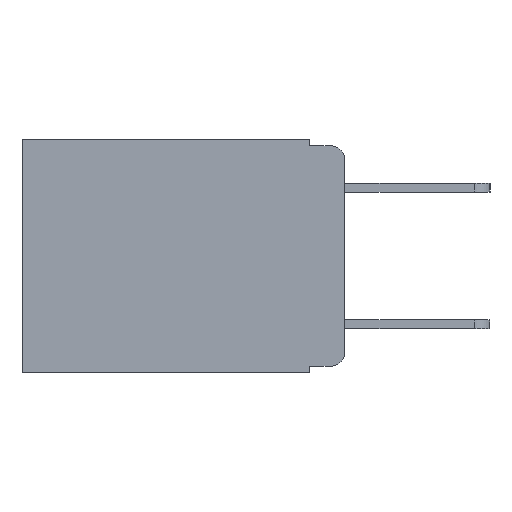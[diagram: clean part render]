
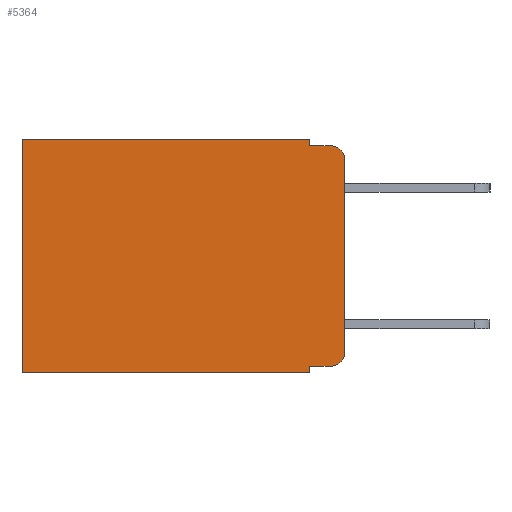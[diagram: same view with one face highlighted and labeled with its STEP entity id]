
A CAD part, left-side view. The second image highlights one B-rep face of the part: STEP entity #5364.
In plain terms, the highlighted planar face has unit normal (-1, 0, 0).
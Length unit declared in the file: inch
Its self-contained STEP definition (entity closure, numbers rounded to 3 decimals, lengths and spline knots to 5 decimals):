
#39 = CARTESIAN_POINT ( 'NONE',  ( 0.298, 0.02, -0.03 ) ) ;
#48 = DIRECTION ( 'NONE',  ( 0., 0., -1. ) ) ;
#63 = VECTOR ( 'NONE', #7219, 39.37008 ) ;
#110 = CARTESIAN_POINT ( 'NONE',  ( 0.298, 0.051, 0. ) ) ;
#261 = ORIENTED_EDGE ( 'NONE', *, *, #4101, .T. ) ;
#610 = CARTESIAN_POINT ( 'NONE',  ( 0.298, 0.051, 0. ) ) ;
#1132 = EDGE_CURVE ( 'NONE', #8445, #1394, #11662, .T. ) ;
#1369 = VERTEX_POINT ( 'NONE', #3259 ) ;
#1370 = EDGE_CURVE ( 'NONE', #6006, #1394, #7896, .T. ) ;
#1394 = VERTEX_POINT ( 'NONE', #6866 ) ;
#1484 = LINE ( 'NONE', #9484, #6356 ) ;
#1754 = CARTESIAN_POINT ( 'NONE',  ( 0.298, 0.051, -0.333 ) ) ;
#1926 = CARTESIAN_POINT ( 'NONE',  ( 0.298, 0., -0.03 ) ) ;
#1969 = DIRECTION ( 'NONE',  ( -1., 0., 0. ) ) ;
#2356 = VERTEX_POINT ( 'NONE', #8151 ) ;
#2420 = DIRECTION ( 'NONE',  ( 0., 0., -1. ) ) ;
#2481 = CARTESIAN_POINT ( 'NONE',  ( 0.298, 0.051, -0.333 ) ) ;
#2482 = DIRECTION ( 'NONE',  ( 0., 0., -1. ) ) ;
#2542 = DIRECTION ( 'NONE',  ( 0., 0., -1. ) ) ;
#2548 = CARTESIAN_POINT ( 'NONE',  ( 0.298, 0.051, -0.343 ) ) ;
#2586 = AXIS2_PLACEMENT_3D ( 'NONE', #3926, #7556, #2420 ) ;
#2650 = DIRECTION ( 'NONE',  ( 0., 0., -1. ) ) ;
#2749 = EDGE_LOOP ( 'NONE', ( #3449, #7786, #8917, #2861, #9144, #10350, #8103, #8748, #261, #3269 ) ) ;
#2774 = CARTESIAN_POINT ( 'NONE',  ( 0.298, 0.473, 0. ) ) ;
#2861 = ORIENTED_EDGE ( 'NONE', *, *, #6523, .F. ) ;
#3032 = CARTESIAN_POINT ( 'NONE',  ( 0.298, 0.02, -0.313 ) ) ;
#3047 = LINE ( 'NONE', #610, #10782 ) ;
#3259 = CARTESIAN_POINT ( 'NONE',  ( 0.298, 0.02, -0.01 ) ) ;
#3260 = VECTOR ( 'NONE', #10368, 39.37008 ) ;
#3269 = ORIENTED_EDGE ( 'NONE', *, *, #1132, .T. ) ;
#3314 = CARTESIAN_POINT ( 'NONE',  ( 0.298, 0.051, 0. ) ) ;
#3449 = ORIENTED_EDGE ( 'NONE', *, *, #1370, .F. ) ;
#3595 = AXIS2_PLACEMENT_3D ( 'NONE', #39, #1969, #9251 ) ;
#3722 = LINE ( 'NONE', #110, #10952 ) ;
#3926 = CARTESIAN_POINT ( 'NONE',  ( 0.298, 0., 0. ) ) ;
#4101 = EDGE_CURVE ( 'NONE', #10851, #8445, #7963, .T. ) ;
#4497 = LINE ( 'NONE', #11727, #63 ) ;
#4716 = EDGE_CURVE ( 'NONE', #11555, #2356, #4497, .T. ) ;
#4819 = DIRECTION ( 'NONE',  ( 0., 0., -1. ) ) ;
#4927 = EDGE_CURVE ( 'NONE', #7244, #1369, #1484, .T. ) ;
#5047 = CARTESIAN_POINT ( 'NONE',  ( 0.298, 0., 0. ) ) ;
#5228 = FACE_OUTER_BOUND ( 'NONE', #2749, .T. ) ;
#5263 = EDGE_CURVE ( 'NONE', #10851, #11555, #3047, .T. ) ;
#5319 = CIRCLE ( 'NONE', #3595, 0.02 ) ;
#5343 = LINE ( 'NONE', #11486, #8007 ) ;
#5364 = ADVANCED_FACE ( 'NONE', ( #5228 ), #11501, .F. ) ;
#5790 = VECTOR ( 'NONE', #2482, 39.37008 ) ;
#5970 = AXIS2_PLACEMENT_3D ( 'NONE', #3032, #11044, #4819 ) ;
#6006 = VERTEX_POINT ( 'NONE', #1926 ) ;
#6356 = VECTOR ( 'NONE', #8579, 39.37008 ) ;
#6523 = EDGE_CURVE ( 'NONE', #8996, #7244, #3722, .T. ) ;
#6866 = CARTESIAN_POINT ( 'NONE',  ( 0.298, 0., -0.313 ) ) ;
#7219 = DIRECTION ( 'NONE',  ( 0., 1., 0. ) ) ;
#7244 = VERTEX_POINT ( 'NONE', #9757 ) ;
#7556 = DIRECTION ( 'NONE',  ( 1., 0., 0. ) ) ;
#7786 = ORIENTED_EDGE ( 'NONE', *, *, #8191, .T. ) ;
#7896 = LINE ( 'NONE', #5047, #5790 ) ;
#7963 = LINE ( 'NONE', #2481, #10006 ) ;
#8007 = VECTOR ( 'NONE', #2650, 39.37008 ) ;
#8103 = ORIENTED_EDGE ( 'NONE', *, *, #4716, .F. ) ;
#8151 = CARTESIAN_POINT ( 'NONE',  ( 0.298, 0.473, -0.343 ) ) ;
#8191 = EDGE_CURVE ( 'NONE', #6006, #1369, #5319, .T. ) ;
#8445 = VERTEX_POINT ( 'NONE', #10704 ) ;
#8532 = CARTESIAN_POINT ( 'NONE',  ( 0.298, 0., 0. ) ) ;
#8579 = DIRECTION ( 'NONE',  ( 0., -1., 0. ) ) ;
#8748 = ORIENTED_EDGE ( 'NONE', *, *, #5263, .F. ) ;
#8794 = DIRECTION ( 'NONE',  ( 0., -1., 0. ) ) ;
#8917 = ORIENTED_EDGE ( 'NONE', *, *, #4927, .F. ) ;
#8996 = VERTEX_POINT ( 'NONE', #3314 ) ;
#9144 = ORIENTED_EDGE ( 'NONE', *, *, #11016, .T. ) ;
#9251 = DIRECTION ( 'NONE',  ( 0., 0., -1. ) ) ;
#9425 = LINE ( 'NONE', #8532, #3260 ) ;
#9440 = VERTEX_POINT ( 'NONE', #2774 ) ;
#9484 = CARTESIAN_POINT ( 'NONE',  ( 0.298, 0.051, -0.01 ) ) ;
#9757 = CARTESIAN_POINT ( 'NONE',  ( 0.298, 0.051, -0.01 ) ) ;
#10006 = VECTOR ( 'NONE', #8794, 39.37008 ) ;
#10350 = ORIENTED_EDGE ( 'NONE', *, *, #10511, .T. ) ;
#10368 = DIRECTION ( 'NONE',  ( 0., 1., 0. ) ) ;
#10511 = EDGE_CURVE ( 'NONE', #9440, #2356, #5343, .T. ) ;
#10704 = CARTESIAN_POINT ( 'NONE',  ( 0.298, 0.02, -0.333 ) ) ;
#10782 = VECTOR ( 'NONE', #2542, 39.37008 ) ;
#10851 = VERTEX_POINT ( 'NONE', #1754 ) ;
#10952 = VECTOR ( 'NONE', #48, 39.37008 ) ;
#11016 = EDGE_CURVE ( 'NONE', #8996, #9440, #9425, .T. ) ;
#11044 = DIRECTION ( 'NONE',  ( -1., 0., 0. ) ) ;
#11486 = CARTESIAN_POINT ( 'NONE',  ( 0.298, 0.473, 0. ) ) ;
#11501 = PLANE ( 'NONE',  #2586 ) ;
#11555 = VERTEX_POINT ( 'NONE', #2548 ) ;
#11662 = CIRCLE ( 'NONE', #5970, 0.02 ) ;
#11727 = CARTESIAN_POINT ( 'NONE',  ( 0.298, 0., -0.343 ) ) ;
